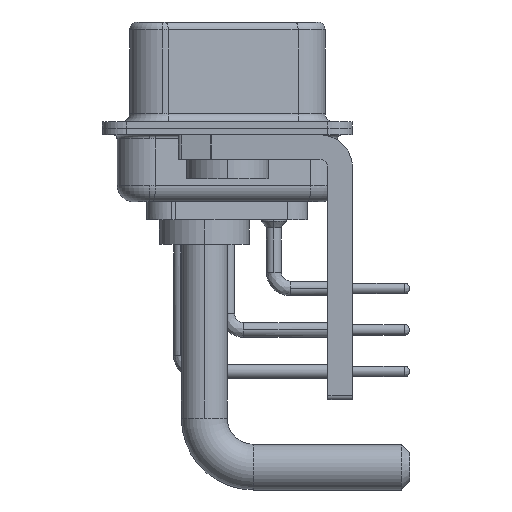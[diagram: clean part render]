
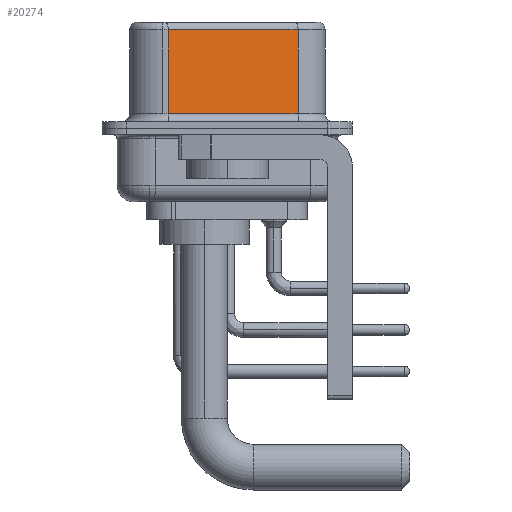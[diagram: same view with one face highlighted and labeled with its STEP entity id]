
A CAD part, left-side view. The second image highlights one B-rep face of the part: STEP entity #20274.
In plain terms, the highlighted planar face has unit normal (-0.985, -0.174, 0).
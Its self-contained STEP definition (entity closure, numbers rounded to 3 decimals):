
#1342 = CARTESIAN_POINT ( 'NONE',  ( 5.132, -4.322, 0.9 ) ) ;
#1416 = ORIENTED_EDGE ( 'NONE', *, *, #4175, .T. ) ;
#1866 = LINE ( 'NONE', #9689, #4636 ) ;
#2945 = VERTEX_POINT ( 'NONE', #29255 ) ;
#4175 = EDGE_CURVE ( 'NONE', #23734, #21641, #16242, .T. ) ;
#4636 = VECTOR ( 'NONE', #20720, 1000. ) ;
#4829 = ORIENTED_EDGE ( 'NONE', *, *, #13859, .T. ) ;
#5206 = CARTESIAN_POINT ( 'NONE',  ( 5.132, -4.322, 0.9 ) ) ;
#6199 = DIRECTION ( 'NONE',  ( -0.174, 0.985, 0. ) ) ;
#8525 = CARTESIAN_POINT ( 'NONE',  ( 5.132, -4.322, 6.52 ) ) ;
#9689 = CARTESIAN_POINT ( 'NONE',  ( 5.132, -4.322, 6.52 ) ) ;
#10399 = CARTESIAN_POINT ( 'NONE',  ( 3.73, 3.628, 6.52 ) ) ;
#11719 = PLANE ( 'NONE',  #12942 ) ;
#12316 = CARTESIAN_POINT ( 'NONE',  ( 5.132, -4.322, 6.02 ) ) ;
#12644 = ORIENTED_EDGE ( 'NONE', *, *, #25825, .F. ) ;
#12942 = AXIS2_PLACEMENT_3D ( 'NONE', #8525, #27559, #6199 ) ;
#13859 = EDGE_CURVE ( 'NONE', #21641, #30969, #29577, .T. ) ;
#15145 = DIRECTION ( 'NONE',  ( -0.174, 0.985, 0. ) ) ;
#16242 = LINE ( 'NONE', #10399, #30658 ) ;
#18923 = DIRECTION ( 'NONE',  ( 0., 0., -1. ) ) ;
#19883 = FACE_OUTER_BOUND ( 'NONE', #21006, .T. ) ;
#20274 = ADVANCED_FACE ( 'NONE', ( #19883 ), #11719, .F. ) ;
#20720 = DIRECTION ( 'NONE',  ( 0., 0., -1. ) ) ;
#21006 = EDGE_LOOP ( 'NONE', ( #12644, #29933, #1416, #4829 ) ) ;
#21641 = VERTEX_POINT ( 'NONE', #27075 ) ;
#23734 = VERTEX_POINT ( 'NONE', #29338 ) ;
#25825 = EDGE_CURVE ( 'NONE', #2945, #30969, #1866, .T. ) ;
#27075 = CARTESIAN_POINT ( 'NONE',  ( 3.73, 3.628, 0.9 ) ) ;
#27559 = DIRECTION ( 'NONE',  ( 0.985, 0.174, 0. ) ) ;
#27887 = EDGE_CURVE ( 'NONE', #2945, #23734, #28697, .T. ) ;
#28021 = VECTOR ( 'NONE', #28577, 1000. ) ;
#28577 = DIRECTION ( 'NONE',  ( 0.174, -0.985, 0. ) ) ;
#28697 = LINE ( 'NONE', #12316, #32639 ) ;
#29255 = CARTESIAN_POINT ( 'NONE',  ( 5.132, -4.322, 6.02 ) ) ;
#29338 = CARTESIAN_POINT ( 'NONE',  ( 3.73, 3.628, 6.02 ) ) ;
#29577 = LINE ( 'NONE', #5206, #28021 ) ;
#29933 = ORIENTED_EDGE ( 'NONE', *, *, #27887, .T. ) ;
#30658 = VECTOR ( 'NONE', #18923, 1000. ) ;
#30969 = VERTEX_POINT ( 'NONE', #1342 ) ;
#32639 = VECTOR ( 'NONE', #15145, 1000. ) ;
